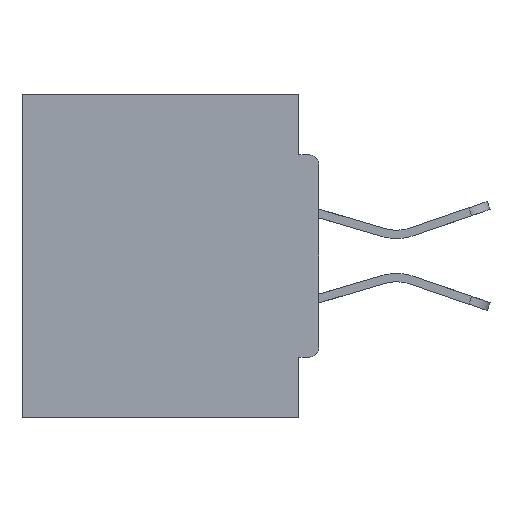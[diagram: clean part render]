
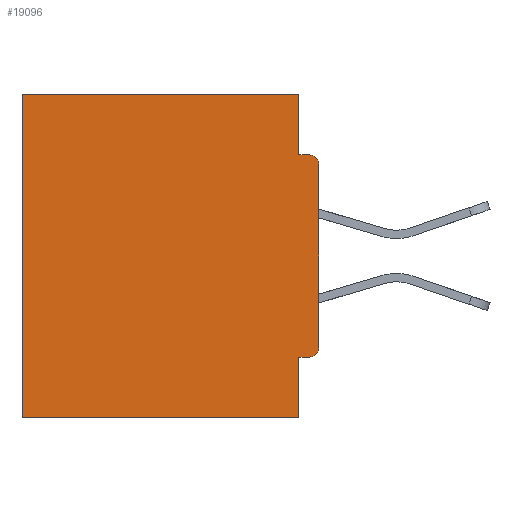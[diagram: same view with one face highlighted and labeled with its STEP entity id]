
A CAD part, left-side view. The second image highlights one B-rep face of the part: STEP entity #19096.
In plain terms, the highlighted planar face has unit normal (-1, 0, 0).
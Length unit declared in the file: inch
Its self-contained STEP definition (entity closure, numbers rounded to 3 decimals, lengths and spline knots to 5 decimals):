
#624 = DIRECTION ( 'NONE',  ( -1., 0., 0. ) ) ;
#1098 = CARTESIAN_POINT ( 'NONE',  ( 0.298, 0.031, -0.5 ) ) ;
#1310 = VERTEX_POINT ( 'NONE', #33153 ) ;
#1351 = DIRECTION ( 'NONE',  ( 0., 1., 0. ) ) ;
#1360 = ORIENTED_EDGE ( 'NONE', *, *, #30647, .F. ) ;
#1702 = LINE ( 'NONE', #35411, #13021 ) ;
#1963 = LINE ( 'NONE', #20120, #5023 ) ;
#2402 = DIRECTION ( 'NONE',  ( 0., 0., -1. ) ) ;
#2543 = CARTESIAN_POINT ( 'NONE',  ( 0.298, 0.46, 0. ) ) ;
#2646 = CARTESIAN_POINT ( 'NONE',  ( 0.298, 0., 0. ) ) ;
#2726 = EDGE_CURVE ( 'NONE', #30224, #4403, #11978, .T. ) ;
#3340 = EDGE_CURVE ( 'NONE', #31794, #20374, #36034, .T. ) ;
#3722 = ORIENTED_EDGE ( 'NONE', *, *, #31605, .F. ) ;
#4403 = VERTEX_POINT ( 'NONE', #23796 ) ;
#4446 = DIRECTION ( 'NONE',  ( 0., 0., -1. ) ) ;
#5023 = VECTOR ( 'NONE', #34318, 39.37008 ) ;
#5080 = EDGE_CURVE ( 'NONE', #27104, #31794, #7482, .T. ) ;
#5437 = VERTEX_POINT ( 'NONE', #30211 ) ;
#5628 = EDGE_LOOP ( 'NONE', ( #29414, #8309, #27328, #33599, #25301, #1360, #3722, #20663, #26456, #15402 ) ) ;
#7296 = VERTEX_POINT ( 'NONE', #30380 ) ;
#7396 = DIRECTION ( 'NONE',  ( 0., 0., -1. ) ) ;
#7429 = VERTEX_POINT ( 'NONE', #31244 ) ;
#7482 = LINE ( 'NONE', #15375, #24570 ) ;
#7733 = VERTEX_POINT ( 'NONE', #23521 ) ;
#8309 = ORIENTED_EDGE ( 'NONE', *, *, #31418, .F. ) ;
#8914 = CARTESIAN_POINT ( 'NONE',  ( 0.298, 0.015, -0.3915 ) ) ;
#9169 = DIRECTION ( 'NONE',  ( 0., 1., 0. ) ) ;
#9774 = EDGE_CURVE ( 'NONE', #27104, #7296, #28689, .T. ) ;
#9893 = VECTOR ( 'NONE', #10711, 39.37008 ) ;
#10433 = EDGE_CURVE ( 'NONE', #7429, #1310, #11201, .T. ) ;
#10711 = DIRECTION ( 'NONE',  ( 0., 1., 0. ) ) ;
#11201 = CIRCLE ( 'NONE', #33888, 0.015 ) ;
#11619 = CARTESIAN_POINT ( 'NONE',  ( 0.298, 0.015, -0.4065 ) ) ;
#11978 = CIRCLE ( 'NONE', #29688, 0.015 ) ;
#12651 = LINE ( 'NONE', #14759, #34134 ) ;
#13021 = VECTOR ( 'NONE', #7396, 39.37008 ) ;
#13734 = PLANE ( 'NONE',  #30523 ) ;
#14759 = CARTESIAN_POINT ( 'NONE',  ( 0.298, 0., -0.5 ) ) ;
#15105 = LINE ( 'NONE', #30238, #9893 ) ;
#15375 = CARTESIAN_POINT ( 'NONE',  ( 0.298, 0., 0. ) ) ;
#15402 = ORIENTED_EDGE ( 'NONE', *, *, #17741, .F. ) ;
#15668 = LINE ( 'NONE', #23308, #18750 ) ;
#16499 = CARTESIAN_POINT ( 'NONE',  ( 0.298, 0.46, 0. ) ) ;
#16871 = DIRECTION ( 'NONE',  ( 0., 0., -1. ) ) ;
#17658 = CARTESIAN_POINT ( 'NONE',  ( 0.298, 0.031, 0. ) ) ;
#17741 = EDGE_CURVE ( 'NONE', #7429, #4403, #1963, .T. ) ;
#18750 = VECTOR ( 'NONE', #26464, 39.37008 ) ;
#19096 = ADVANCED_FACE ( 'NONE', ( #33373 ), #13734, .F. ) ;
#19975 = VECTOR ( 'NONE', #20722, 39.37008 ) ;
#20120 = CARTESIAN_POINT ( 'NONE',  ( 0.298, 0., 0. ) ) ;
#20374 = VERTEX_POINT ( 'NONE', #32271 ) ;
#20663 = ORIENTED_EDGE ( 'NONE', *, *, #24455, .F. ) ;
#20722 = DIRECTION ( 'NONE',  ( 0., 0., -1. ) ) ;
#23308 = CARTESIAN_POINT ( 'NONE',  ( 0.298, 0., -0.0935 ) ) ;
#23521 = CARTESIAN_POINT ( 'NONE',  ( 0.298, 0.031, -0.4065 ) ) ;
#23796 = CARTESIAN_POINT ( 'NONE',  ( 0.298, 0., -0.3915 ) ) ;
#24455 = EDGE_CURVE ( 'NONE', #30224, #7733, #15105, .T. ) ;
#24570 = VECTOR ( 'NONE', #1351, 39.37008 ) ;
#24839 = DIRECTION ( 'NONE',  ( -1., 0., 0. ) ) ;
#24856 = DIRECTION ( 'NONE',  ( 1., 0., 0. ) ) ;
#25301 = ORIENTED_EDGE ( 'NONE', *, *, #3340, .T. ) ;
#26386 = VECTOR ( 'NONE', #16871, 39.37008 ) ;
#26456 = ORIENTED_EDGE ( 'NONE', *, *, #2726, .T. ) ;
#26464 = DIRECTION ( 'NONE',  ( 0., -1., 0. ) ) ;
#27104 = VERTEX_POINT ( 'NONE', #17658 ) ;
#27328 = ORIENTED_EDGE ( 'NONE', *, *, #9774, .F. ) ;
#27373 = CARTESIAN_POINT ( 'NONE',  ( 0.298, 0.015, -0.1085 ) ) ;
#28689 = LINE ( 'NONE', #1098, #19975 ) ;
#29414 = ORIENTED_EDGE ( 'NONE', *, *, #10433, .T. ) ;
#29688 = AXIS2_PLACEMENT_3D ( 'NONE', #8914, #624, #4446 ) ;
#30211 = CARTESIAN_POINT ( 'NONE',  ( 0.298, 0.031, -0.5 ) ) ;
#30224 = VERTEX_POINT ( 'NONE', #11619 ) ;
#30238 = CARTESIAN_POINT ( 'NONE',  ( 0.298, 0., -0.4065 ) ) ;
#30380 = CARTESIAN_POINT ( 'NONE',  ( 0.298, 0.031, -0.0935 ) ) ;
#30523 = AXIS2_PLACEMENT_3D ( 'NONE', #2646, #24856, #2402 ) ;
#30647 = EDGE_CURVE ( 'NONE', #5437, #20374, #12651, .T. ) ;
#31244 = CARTESIAN_POINT ( 'NONE',  ( 0.298, 0., -0.1085 ) ) ;
#31418 = EDGE_CURVE ( 'NONE', #7296, #1310, #15668, .T. ) ;
#31605 = EDGE_CURVE ( 'NONE', #7733, #5437, #1702, .T. ) ;
#31794 = VERTEX_POINT ( 'NONE', #2543 ) ;
#32271 = CARTESIAN_POINT ( 'NONE',  ( 0.298, 0.46, -0.5 ) ) ;
#33024 = DIRECTION ( 'NONE',  ( 0., 0., -1. ) ) ;
#33153 = CARTESIAN_POINT ( 'NONE',  ( 0.298, 0.015, -0.0935 ) ) ;
#33373 = FACE_OUTER_BOUND ( 'NONE', #5628, .T. ) ;
#33599 = ORIENTED_EDGE ( 'NONE', *, *, #5080, .T. ) ;
#33888 = AXIS2_PLACEMENT_3D ( 'NONE', #27373, #24839, #33024 ) ;
#34134 = VECTOR ( 'NONE', #9169, 39.37008 ) ;
#34318 = DIRECTION ( 'NONE',  ( 0., 0., -1. ) ) ;
#35411 = CARTESIAN_POINT ( 'NONE',  ( 0.298, 0.031, -0.5 ) ) ;
#36034 = LINE ( 'NONE', #16499, #26386 ) ;
